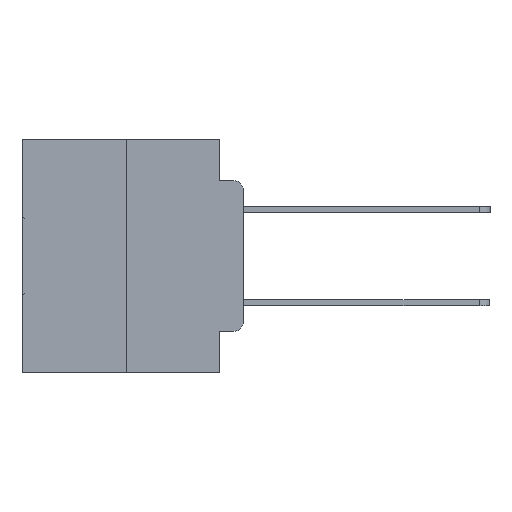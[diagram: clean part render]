
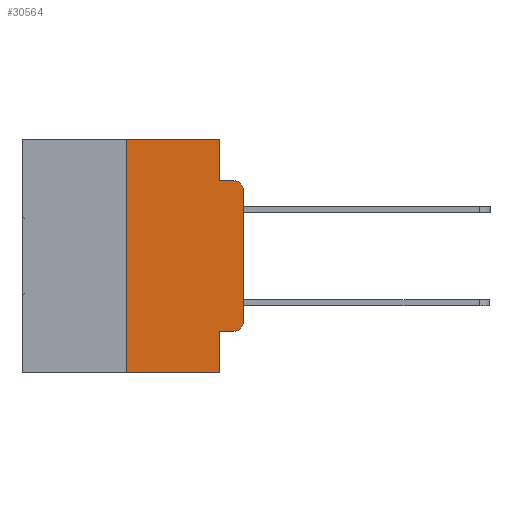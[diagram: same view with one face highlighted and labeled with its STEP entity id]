
A CAD part, left-side view. The second image highlights one B-rep face of the part: STEP entity #30564.
In plain terms, the highlighted planar face has unit normal (-1, 0, 0).
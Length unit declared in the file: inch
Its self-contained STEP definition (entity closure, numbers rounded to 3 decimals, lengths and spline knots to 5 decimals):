
#128 = LINE ( 'NONE', #10314, #6800 ) ;
#426 = VECTOR ( 'NONE', #15933, 39.37008 ) ;
#893 = EDGE_LOOP ( 'NONE', ( #2430, #11083, #8720, #28472, #1646, #3232, #7864, #10361, #1559, #26061 ) ) ;
#1164 = VERTEX_POINT ( 'NONE', #13194 ) ;
#1559 = ORIENTED_EDGE ( 'NONE', *, *, #14863, .T. ) ;
#1646 = ORIENTED_EDGE ( 'NONE', *, *, #27382, .F. ) ;
#1660 = CARTESIAN_POINT ( 'NONE',  ( 0., 0.473, 0. ) ) ;
#2187 = EDGE_CURVE ( 'NONE', #20351, #32292, #15234, .T. ) ;
#2430 = ORIENTED_EDGE ( 'NONE', *, *, #12343, .T. ) ;
#2493 = CARTESIAN_POINT ( 'NONE',  ( 0., 0.051, -0.5 ) ) ;
#2736 = DIRECTION ( 'NONE',  ( -1., 0., 0. ) ) ;
#3048 = VERTEX_POINT ( 'NONE', #29725 ) ;
#3232 = ORIENTED_EDGE ( 'NONE', *, *, #29829, .F. ) ;
#3462 = CARTESIAN_POINT ( 'NONE',  ( 0., 0.473, 0. ) ) ;
#3800 = CARTESIAN_POINT ( 'NONE',  ( 0., 0.051, 0. ) ) ;
#3892 = CARTESIAN_POINT ( 'NONE',  ( 0., 0.051, -0.4115 ) ) ;
#4177 = DIRECTION ( 'NONE',  ( 0., -1., 0. ) ) ;
#4798 = VECTOR ( 'NONE', #30730, 39.37008 ) ;
#5525 = VERTEX_POINT ( 'NONE', #13905 ) ;
#5972 = DIRECTION ( 'NONE',  ( 1., 0., 0. ) ) ;
#6380 = CARTESIAN_POINT ( 'NONE',  ( 0., 0.02, -0.3915 ) ) ;
#6800 = VECTOR ( 'NONE', #25470, 39.37008 ) ;
#7024 = EDGE_CURVE ( 'NONE', #7044, #1164, #25212, .T. ) ;
#7044 = VERTEX_POINT ( 'NONE', #10231 ) ;
#7079 = CARTESIAN_POINT ( 'NONE',  ( 0., 0.051, 0. ) ) ;
#7099 = LINE ( 'NONE', #25924, #426 ) ;
#7750 = EDGE_CURVE ( 'NONE', #3048, #1164, #32461, .T. ) ;
#7864 = ORIENTED_EDGE ( 'NONE', *, *, #18482, .T. ) ;
#8460 = VECTOR ( 'NONE', #31512, 39.37008 ) ;
#8720 = ORIENTED_EDGE ( 'NONE', *, *, #7750, .F. ) ;
#8945 = DIRECTION ( 'NONE',  ( 0., 0., -1. ) ) ;
#9547 = EDGE_CURVE ( 'NONE', #12402, #5525, #14575, .T. ) ;
#10231 = CARTESIAN_POINT ( 'NONE',  ( 0., 0., -0.1085 ) ) ;
#10314 = CARTESIAN_POINT ( 'NONE',  ( 0., 0., 0. ) ) ;
#10361 = ORIENTED_EDGE ( 'NONE', *, *, #2187, .F. ) ;
#10517 = CARTESIAN_POINT ( 'NONE',  ( 0., 0.02, -0.4115 ) ) ;
#10624 = CARTESIAN_POINT ( 'NONE',  ( 0., 0.051, -0.0885 ) ) ;
#10746 = EDGE_CURVE ( 'NONE', #10940, #3048, #21976, .T. ) ;
#10924 = LINE ( 'NONE', #21516, #17701 ) ;
#10940 = VERTEX_POINT ( 'NONE', #7079 ) ;
#11083 = ORIENTED_EDGE ( 'NONE', *, *, #7024, .T. ) ;
#11491 = VECTOR ( 'NONE', #28302, 39.37008 ) ;
#12334 = LINE ( 'NONE', #28167, #4798 ) ;
#12343 = EDGE_CURVE ( 'NONE', #5525, #7044, #128, .T. ) ;
#12402 = VERTEX_POINT ( 'NONE', #10517 ) ;
#13194 = CARTESIAN_POINT ( 'NONE',  ( 0., 0.02, -0.0885 ) ) ;
#13659 = LINE ( 'NONE', #1660, #27067 ) ;
#13905 = CARTESIAN_POINT ( 'NONE',  ( 0., 0., -0.3915 ) ) ;
#14013 = DIRECTION ( 'NONE',  ( 0., 0., -1. ) ) ;
#14073 = CARTESIAN_POINT ( 'NONE',  ( 0., 0.051, 0. ) ) ;
#14575 = CIRCLE ( 'NONE', #21557, 0.02 ) ;
#14760 = AXIS2_PLACEMENT_3D ( 'NONE', #17913, #2736, #20421 ) ;
#14863 = EDGE_CURVE ( 'NONE', #20351, #12402, #12334, .T. ) ;
#15234 = LINE ( 'NONE', #14073, #8460 ) ;
#15269 = VECTOR ( 'NONE', #14013, 39.37008 ) ;
#15933 = DIRECTION ( 'NONE',  ( 0., 0., 1. ) ) ;
#16165 = CARTESIAN_POINT ( 'NONE',  ( 0., 0.25, -0.5 ) ) ;
#17701 = VECTOR ( 'NONE', #24033, 39.37008 ) ;
#17913 = CARTESIAN_POINT ( 'NONE',  ( 0., 0.02, -0.1085 ) ) ;
#18281 = CARTESIAN_POINT ( 'NONE',  ( 0., 0.25, 0. ) ) ;
#18482 = EDGE_CURVE ( 'NONE', #22862, #32292, #10924, .T. ) ;
#18647 = PLANE ( 'NONE',  #27736 ) ;
#18947 = VERTEX_POINT ( 'NONE', #18281 ) ;
#19808 = FACE_OUTER_BOUND ( 'NONE', #893, .T. ) ;
#20351 = VERTEX_POINT ( 'NONE', #3892 ) ;
#20421 = DIRECTION ( 'NONE',  ( 0., 0., -1. ) ) ;
#21516 = CARTESIAN_POINT ( 'NONE',  ( 0., 0.473, -0.5 ) ) ;
#21557 = AXIS2_PLACEMENT_3D ( 'NONE', #6380, #24125, #8945 ) ;
#21976 = LINE ( 'NONE', #3800, #15269 ) ;
#22862 = VERTEX_POINT ( 'NONE', #16165 ) ;
#23717 = DIRECTION ( 'NONE',  ( 0., 0., -1. ) ) ;
#24033 = DIRECTION ( 'NONE',  ( 0., -1., 0. ) ) ;
#24125 = DIRECTION ( 'NONE',  ( -1., 0., 0. ) ) ;
#25212 = CIRCLE ( 'NONE', #14760, 0.02 ) ;
#25470 = DIRECTION ( 'NONE',  ( 0., 0., 1. ) ) ;
#25924 = CARTESIAN_POINT ( 'NONE',  ( 0., 0.25, 0. ) ) ;
#26061 = ORIENTED_EDGE ( 'NONE', *, *, #9547, .T. ) ;
#27067 = VECTOR ( 'NONE', #4177, 39.37008 ) ;
#27382 = EDGE_CURVE ( 'NONE', #18947, #10940, #13659, .T. ) ;
#27736 = AXIS2_PLACEMENT_3D ( 'NONE', #3462, #5972, #23717 ) ;
#28167 = CARTESIAN_POINT ( 'NONE',  ( 0., 0.051, -0.4115 ) ) ;
#28302 = DIRECTION ( 'NONE',  ( 0., -1., 0. ) ) ;
#28472 = ORIENTED_EDGE ( 'NONE', *, *, #10746, .F. ) ;
#29725 = CARTESIAN_POINT ( 'NONE',  ( 0., 0.051, -0.0885 ) ) ;
#29829 = EDGE_CURVE ( 'NONE', #22862, #18947, #7099, .T. ) ;
#30564 = ADVANCED_FACE ( 'NONE', ( #19808 ), #18647, .F. ) ;
#30730 = DIRECTION ( 'NONE',  ( 0., -1., 0. ) ) ;
#31512 = DIRECTION ( 'NONE',  ( 0., 0., -1. ) ) ;
#32292 = VERTEX_POINT ( 'NONE', #2493 ) ;
#32461 = LINE ( 'NONE', #10624, #11491 ) ;
